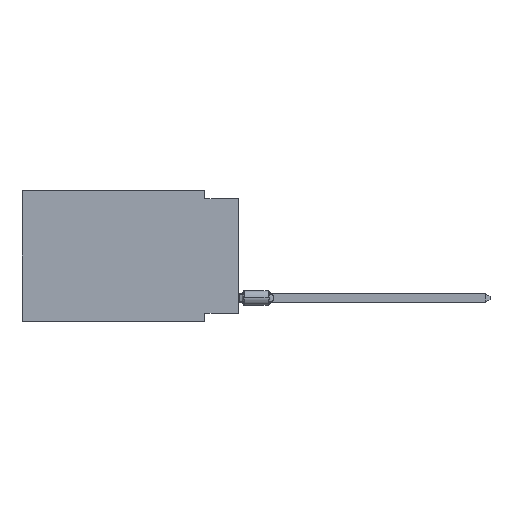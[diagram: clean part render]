
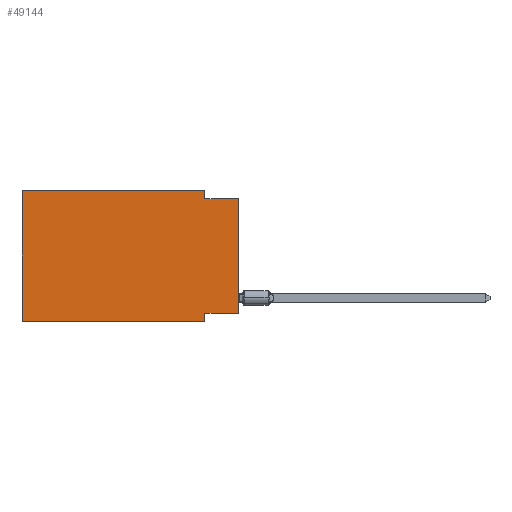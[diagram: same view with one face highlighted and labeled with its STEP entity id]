
A CAD part, left-side view. The second image highlights one B-rep face of the part: STEP entity #49144.
In plain terms, the highlighted planar face has unit normal (-1, 0, 0).
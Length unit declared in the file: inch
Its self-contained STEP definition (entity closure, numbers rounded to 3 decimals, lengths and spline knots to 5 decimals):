
#1924 = LINE ( 'NONE', #14227, #78211 ) ;
#2329 = LINE ( 'NONE', #26525, #16817 ) ;
#2531 = CARTESIAN_POINT ( 'NONE',  ( 0., 0.1, -0.365 ) ) ;
#2558 = CARTESIAN_POINT ( 'NONE',  ( 0., 0.1, 0. ) ) ;
#3283 = VERTEX_POINT ( 'NONE', #19115 ) ;
#3795 = EDGE_CURVE ( 'NONE', #13865, #59343, #1924, .T. ) ;
#3839 = VECTOR ( 'NONE', #27711, 39.37008 ) ;
#4279 = ORIENTED_EDGE ( 'NONE', *, *, #70337, .F. ) ;
#6675 = VECTOR ( 'NONE', #47629, 39.37008 ) ;
#9311 = CARTESIAN_POINT ( 'NONE',  ( 0., 0.1, -0.39 ) ) ;
#9440 = DIRECTION ( 'NONE',  ( 0., 0., 1. ) ) ;
#10159 = EDGE_CURVE ( 'NONE', #13865, #61688, #10617, .T. ) ;
#10617 = LINE ( 'NONE', #28476, #3839 ) ;
#12056 = EDGE_CURVE ( 'NONE', #17203, #59343, #22910, .T. ) ;
#12337 = PLANE ( 'NONE',  #37031 ) ;
#13170 = EDGE_CURVE ( 'NONE', #58885, #13570, #2329, .T. ) ;
#13570 = VERTEX_POINT ( 'NONE', #20494 ) ;
#13865 = VERTEX_POINT ( 'NONE', #31124 ) ;
#14227 = CARTESIAN_POINT ( 'NONE',  ( 0., 0., 0. ) ) ;
#14484 = DIRECTION ( 'NONE',  ( 0., 0., -1. ) ) ;
#14768 = EDGE_CURVE ( 'NONE', #3283, #64031, #34114, .T. ) ;
#15022 = DIRECTION ( 'NONE',  ( 0., -1., 0. ) ) ;
#16817 = VECTOR ( 'NONE', #15022, 39.37008 ) ;
#17203 = VERTEX_POINT ( 'NONE', #23411 ) ;
#17501 = ORIENTED_EDGE ( 'NONE', *, *, #63979, .F. ) ;
#19115 = CARTESIAN_POINT ( 'NONE',  ( 0., 0.645, -0.39 ) ) ;
#20494 = CARTESIAN_POINT ( 'NONE',  ( 0., 0.1, 0. ) ) ;
#22910 = LINE ( 'NONE', #78102, #38245 ) ;
#23411 = CARTESIAN_POINT ( 'NONE',  ( 0., 0.1, -0.025 ) ) ;
#24147 = EDGE_LOOP ( 'NONE', ( #55195, #29630, #17501, #52001, #4279, #49861, #60951, #75877 ) ) ;
#25974 = LINE ( 'NONE', #2558, #44765 ) ;
#26525 = CARTESIAN_POINT ( 'NONE',  ( 0., 0.645, 0. ) ) ;
#27711 = DIRECTION ( 'NONE',  ( 0., 1., 0. ) ) ;
#28476 = CARTESIAN_POINT ( 'NONE',  ( 0., 0., -0.365 ) ) ;
#28629 = VECTOR ( 'NONE', #56438, 39.37008 ) ;
#29248 = DIRECTION ( 'NONE',  ( 0., -1., 0. ) ) ;
#29630 = ORIENTED_EDGE ( 'NONE', *, *, #12056, .F. ) ;
#31124 = CARTESIAN_POINT ( 'NONE',  ( 0., 0., -0.365 ) ) ;
#31552 = DIRECTION ( 'NONE',  ( 0., 0., -1. ) ) ;
#34114 = LINE ( 'NONE', #65499, #6675 ) ;
#36159 = EDGE_CURVE ( 'NONE', #61688, #64031, #57397, .T. ) ;
#36167 = DIRECTION ( 'NONE',  ( 1., 0., 0. ) ) ;
#37031 = AXIS2_PLACEMENT_3D ( 'NONE', #37344, #36167, #54457 ) ;
#37344 = CARTESIAN_POINT ( 'NONE',  ( 0., 0.645, 0. ) ) ;
#38245 = VECTOR ( 'NONE', #29248, 39.37008 ) ;
#38381 = CARTESIAN_POINT ( 'NONE',  ( 0., 0.645, 0. ) ) ;
#44765 = VECTOR ( 'NONE', #31552, 39.37008 ) ;
#47629 = DIRECTION ( 'NONE',  ( 0., -1., 0. ) ) ;
#49144 = ADVANCED_FACE ( 'NONE', ( #60034 ), #12337, .F. ) ;
#49861 = ORIENTED_EDGE ( 'NONE', *, *, #14768, .T. ) ;
#52001 = ORIENTED_EDGE ( 'NONE', *, *, #13170, .F. ) ;
#54457 = DIRECTION ( 'NONE',  ( 0., 0., -1. ) ) ;
#55195 = ORIENTED_EDGE ( 'NONE', *, *, #3795, .T. ) ;
#56438 = DIRECTION ( 'NONE',  ( 0., 0., 1. ) ) ;
#57397 = LINE ( 'NONE', #9311, #70978 ) ;
#58885 = VERTEX_POINT ( 'NONE', #38381 ) ;
#59343 = VERTEX_POINT ( 'NONE', #77182 ) ;
#60034 = FACE_OUTER_BOUND ( 'NONE', #24147, .T. ) ;
#60951 = ORIENTED_EDGE ( 'NONE', *, *, #36159, .F. ) ;
#61386 = CARTESIAN_POINT ( 'NONE',  ( 0., 0.1, -0.39 ) ) ;
#61688 = VERTEX_POINT ( 'NONE', #2531 ) ;
#63979 = EDGE_CURVE ( 'NONE', #13570, #17203, #25974, .T. ) ;
#64031 = VERTEX_POINT ( 'NONE', #61386 ) ;
#65499 = CARTESIAN_POINT ( 'NONE',  ( 0., 0.645, -0.39 ) ) ;
#70337 = EDGE_CURVE ( 'NONE', #3283, #58885, #75091, .T. ) ;
#70978 = VECTOR ( 'NONE', #14484, 39.37008 ) ;
#74294 = CARTESIAN_POINT ( 'NONE',  ( 0., 0.645, 0. ) ) ;
#75091 = LINE ( 'NONE', #74294, #28629 ) ;
#75877 = ORIENTED_EDGE ( 'NONE', *, *, #10159, .F. ) ;
#77182 = CARTESIAN_POINT ( 'NONE',  ( 0., 0., -0.025 ) ) ;
#78102 = CARTESIAN_POINT ( 'NONE',  ( 0., 0., -0.025 ) ) ;
#78211 = VECTOR ( 'NONE', #9440, 39.37008 ) ;
